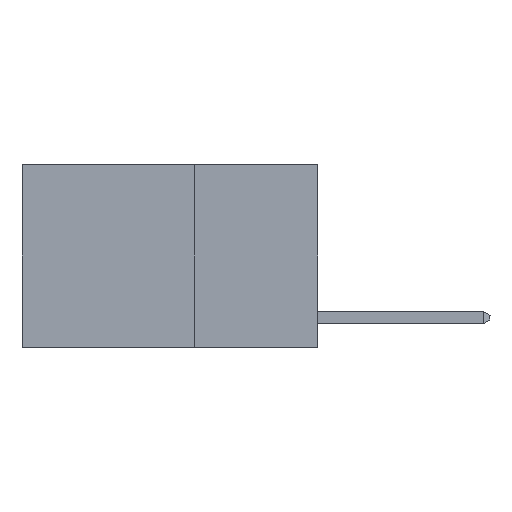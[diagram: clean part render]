
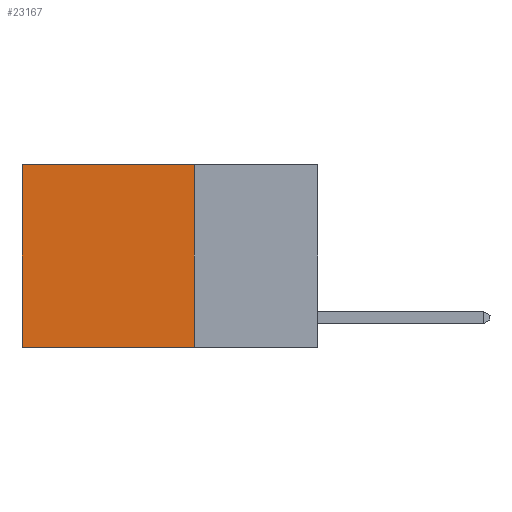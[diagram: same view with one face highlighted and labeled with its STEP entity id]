
A CAD part, left-side view. The second image highlights one B-rep face of the part: STEP entity #23167.
In plain terms, the highlighted planar face has unit normal (-1, 0, 0).
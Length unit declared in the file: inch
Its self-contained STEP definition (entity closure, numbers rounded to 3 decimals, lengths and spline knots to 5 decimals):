
#827 = VERTEX_POINT ( 'NONE', #10539 ) ;
#3025 = LINE ( 'NONE', #24771, #12962 ) ;
#3453 = DIRECTION ( 'NONE',  ( 0., 1., 0. ) ) ;
#5352 = DIRECTION ( 'NONE',  ( 0., 1., 0. ) ) ;
#6509 = ORIENTED_EDGE ( 'NONE', *, *, #23261, .T. ) ;
#6638 = EDGE_CURVE ( 'NONE', #21955, #15721, #26746, .T. ) ;
#7017 = DIRECTION ( 'NONE',  ( 0., 0., -1. ) ) ;
#7543 = EDGE_CURVE ( 'NONE', #15721, #15147, #25084, .T. ) ;
#7871 = CARTESIAN_POINT ( 'NONE',  ( 0.2625, 0.25, -0.37 ) ) ;
#8218 = VECTOR ( 'NONE', #7017, 39.37008 ) ;
#9077 = FACE_OUTER_BOUND ( 'NONE', #26100, .T. ) ;
#10269 = ORIENTED_EDGE ( 'NONE', *, *, #6638, .F. ) ;
#10539 = CARTESIAN_POINT ( 'NONE',  ( 0.2625, 0.6, 0. ) ) ;
#10901 = EDGE_CURVE ( 'NONE', #21955, #827, #3025, .T. ) ;
#11369 = CARTESIAN_POINT ( 'NONE',  ( 0.2625, 0.25, 0. ) ) ;
#11564 = VECTOR ( 'NONE', #11960, 39.37008 ) ;
#11960 = DIRECTION ( 'NONE',  ( 0., 0., -1. ) ) ;
#12962 = VECTOR ( 'NONE', #3453, 39.37008 ) ;
#13832 = PLANE ( 'NONE',  #14321 ) ;
#13980 = DIRECTION ( 'NONE',  ( 1., 0., 0. ) ) ;
#13994 = CARTESIAN_POINT ( 'NONE',  ( 0.2625, 0.6, -0.37 ) ) ;
#14321 = AXIS2_PLACEMENT_3D ( 'NONE', #22740, #13980, #20461 ) ;
#15147 = VERTEX_POINT ( 'NONE', #13994 ) ;
#15721 = VERTEX_POINT ( 'NONE', #7871 ) ;
#16435 = CARTESIAN_POINT ( 'NONE',  ( 0.2625, 0.6, 0. ) ) ;
#18750 = LINE ( 'NONE', #16435, #11564 ) ;
#19590 = ORIENTED_EDGE ( 'NONE', *, *, #7543, .F. ) ;
#20461 = DIRECTION ( 'NONE',  ( 0., 0., -1. ) ) ;
#21158 = VECTOR ( 'NONE', #5352, 39.37008 ) ;
#21935 = ORIENTED_EDGE ( 'NONE', *, *, #10901, .T. ) ;
#21955 = VERTEX_POINT ( 'NONE', #26620 ) ;
#22740 = CARTESIAN_POINT ( 'NONE',  ( 0.2625, 0.25, 0. ) ) ;
#23167 = ADVANCED_FACE ( 'NONE', ( #9077 ), #13832, .F. ) ;
#23261 = EDGE_CURVE ( 'NONE', #827, #15147, #18750, .T. ) ;
#24771 = CARTESIAN_POINT ( 'NONE',  ( 0.2625, 0.25, 0. ) ) ;
#24789 = CARTESIAN_POINT ( 'NONE',  ( 0.2625, 0.25, -0.37 ) ) ;
#25084 = LINE ( 'NONE', #24789, #21158 ) ;
#26100 = EDGE_LOOP ( 'NONE', ( #6509, #19590, #10269, #21935 ) ) ;
#26620 = CARTESIAN_POINT ( 'NONE',  ( 0.2625, 0.25, 0. ) ) ;
#26746 = LINE ( 'NONE', #11369, #8218 ) ;
